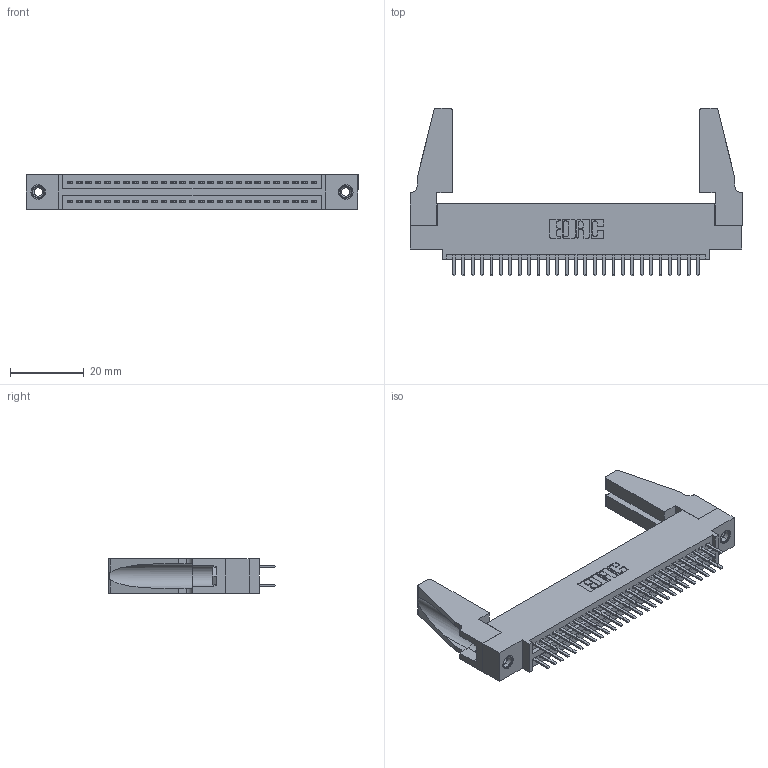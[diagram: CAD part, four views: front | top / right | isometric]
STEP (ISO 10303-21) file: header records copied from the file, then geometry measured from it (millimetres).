
FILE_DESCRIPTION (( 'STEP AP203' ), '1' );
FILE_NAME ('345-054-520-588.STEP', '2019-10-29T18:13:14', ( '' ), ( '' ), 'SwSTEP 2.0', 'SolidWorks 2016', '' );
FILE_SCHEMA (( 'CONFIG_CONTROL_DESIGN' ));
Length unit declared in the file: inch
Products named in the file (5): 345 Part_0.110 Offset - 0.156 Dia-TH; 345-292-001_345-293-120; 345-054-520-588; 345-220-078_345-220-088; 345-250-001_345-250-001-102
Assembly tree (59 placements, depth 2):
  345-054-520-588
    345 Part_0.110 Offset - 0.156 Dia-TH
    345-292-001_345-293-120  x54
    345-250-001_345-250-001-102  x2
    345-220-078_345-220-088  x2
Bounding box: 89.81 x 45.34 x 9.4 mm (x, y, z)
Volume: 11740.8 mm3; surface area: 15421.1 mm2
Topology: 59 solids, 59 shells, 3170 faces, 9145 edges, 5942 vertices
Faces by surface type: plane 2046, cylinder 1108, cone 12, torus 4
Entity records: 25598 total; most frequent: CARTESIAN_POINT 4314, ORIENTED_EDGE 4196, DIRECTION 3814, EDGE_CURVE 2098, VECTOR 1812, LINE 1812, VERTEX_POINT 1390, AXIS2_PLACEMENT_3D 1001
